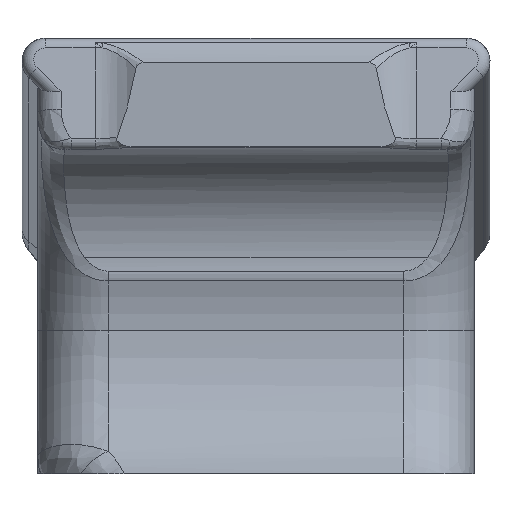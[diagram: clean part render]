
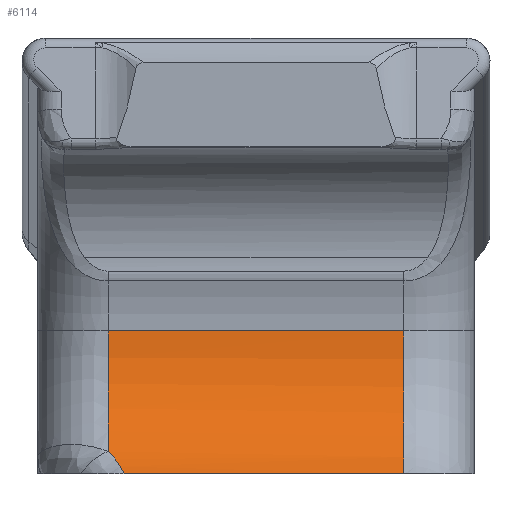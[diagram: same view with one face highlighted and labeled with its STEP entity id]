
A CAD part, left-side view. The second image highlights one B-rep face of the part: STEP entity #6114.
In plain terms, the highlighted cylindrical face has radius 14.287 mm (diameter 28.575 mm), a partial arc.
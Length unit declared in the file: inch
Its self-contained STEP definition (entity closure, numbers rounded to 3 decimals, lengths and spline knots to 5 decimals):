
#129 = CARTESIAN_POINT ( 'NONE',  ( 3.40993, -1.75491, -0.42132 ) ) ;
#167 = CARTESIAN_POINT ( 'NONE',  ( 3.33352, -1.80307, -0.48414 ) ) ;
#827 = B_SPLINE_CURVE_WITH_KNOTS ( 'NONE', 3,
 ( #129, #930, #6098, #1701, #6829, #2431, #7580, #3139, #8293, #3896, #9016, #4653, #167, #5401 ),
 .UNSPECIFIED., .F., .F.,
 ( 4, 2, 2, 1, 1, 2, 2, 4 ),
 ( 0., 0.25, 0.375, 0.4375, 0.46875, 0.48437, 0.5, 1. ),
 .UNSPECIFIED. ) ;
#930 = CARTESIAN_POINT ( 'NONE',  ( 3.40365, -1.76135, -0.42742 ) ) ;
#1022 = DIRECTION ( 'NONE',  ( 0., -1., 0. ) ) ;
#1089 = CARTESIAN_POINT ( 'NONE',  ( 3.31382, -2.74441, -0.49633 ) ) ;
#1487 = CARTESIAN_POINT ( 'NONE',  ( 3.31382, -1.80838, -0.49633 ) ) ;
#1536 = VECTOR ( 'NONE', #5245, 39.37008 ) ;
#1614 = LINE ( 'NONE', #5261, #1536 ) ;
#1629 = CIRCLE ( 'NONE', #3946, 0.5625 ) ;
#1701 = CARTESIAN_POINT ( 'NONE',  ( 3.386, -1.77556, -0.4433 ) ) ;
#1999 = CIRCLE ( 'NONE', #3565, 0.5625 ) ;
#2230 = VECTOR ( 'NONE', #1022, 39.37008 ) ;
#2263 = LINE ( 'NONE', #8339, #2230 ) ;
#2431 = CARTESIAN_POINT ( 'NONE',  ( 3.3764, -1.78195, -0.45141 ) ) ;
#2604 = EDGE_CURVE ( 'NONE', #6706, #9621, #2263, .T. ) ;
#2961 = EDGE_LOOP ( 'NONE', ( #6914, #5644, #6990, #7257, #7335 ) ) ;
#3139 = CARTESIAN_POINT ( 'NONE',  ( 3.36988, -1.78585, -0.45672 ) ) ;
#3213 = CYLINDRICAL_SURFACE ( 'NONE', #5020, 0.5625 ) ;
#3510 = CARTESIAN_POINT ( 'NONE',  ( 3.01782, -1.75491, -0.01801 ) ) ;
#3565 = AXIS2_PLACEMENT_3D ( 'NONE', #4063, #4031, #3993 ) ;
#3582 = EDGE_CURVE ( 'NONE', #6839, #8526, #1614, .T. ) ;
#3896 = CARTESIAN_POINT ( 'NONE',  ( 3.3673, -1.78729, -0.45877 ) ) ;
#3946 = AXIS2_PLACEMENT_3D ( 'NONE', #3510, #8634, #4250 ) ;
#3993 = DIRECTION ( 'NONE',  ( 1., 0., 0. ) ) ;
#4031 = DIRECTION ( 'NONE',  ( 0., -1., 0. ) ) ;
#4063 = CARTESIAN_POINT ( 'NONE',  ( 3.01782, -2.74441, -0.01801 ) ) ;
#4077 = CARTESIAN_POINT ( 'NONE',  ( 3.58032, -2.74441, -0.01801 ) ) ;
#4250 = DIRECTION ( 'NONE',  ( 1., 0., 0. ) ) ;
#4653 = CARTESIAN_POINT ( 'NONE',  ( 3.35092, -1.79623, -0.4717 ) ) ;
#4964 = VERTEX_POINT ( 'NONE', #5832 ) ;
#5020 = AXIS2_PLACEMENT_3D ( 'NONE', #8989, #7674, #7551 ) ;
#5245 = DIRECTION ( 'NONE',  ( 0., 1., 0. ) ) ;
#5261 = CARTESIAN_POINT ( 'NONE',  ( 3.58032, -2.81216, -0.01801 ) ) ;
#5401 = CARTESIAN_POINT ( 'NONE',  ( 3.31382, -1.80838, -0.49633 ) ) ;
#5579 = EDGE_CURVE ( 'NONE', #9621, #6839, #1999, .T. ) ;
#5644 = ORIENTED_EDGE ( 'NONE', *, *, #3582, .T. ) ;
#5832 = CARTESIAN_POINT ( 'NONE',  ( 3.40993, -1.75491, -0.42132 ) ) ;
#6098 = CARTESIAN_POINT ( 'NONE',  ( 3.3969, -1.76732, -0.4337 ) ) ;
#6114 = ADVANCED_FACE ( 'NONE', ( #9201 ), #3213, .F. ) ;
#6706 = VERTEX_POINT ( 'NONE', #1487 ) ;
#6829 = CARTESIAN_POINT ( 'NONE',  ( 3.38224, -1.77818, -0.44653 ) ) ;
#6839 = VERTEX_POINT ( 'NONE', #4077 ) ;
#6914 = ORIENTED_EDGE ( 'NONE', *, *, #5579, .T. ) ;
#6990 = ORIENTED_EDGE ( 'NONE', *, *, #8502, .T. ) ;
#7240 = EDGE_CURVE ( 'NONE', #4964, #6706, #827, .T. ) ;
#7257 = ORIENTED_EDGE ( 'NONE', *, *, #7240, .T. ) ;
#7335 = ORIENTED_EDGE ( 'NONE', *, *, #2604, .T. ) ;
#7551 = DIRECTION ( 'NONE',  ( 1., 0., 0. ) ) ;
#7580 = CARTESIAN_POINT ( 'NONE',  ( 3.37343, -1.78378, -0.45385 ) ) ;
#7674 = DIRECTION ( 'NONE',  ( 0., 1., 0. ) ) ;
#7921 = CARTESIAN_POINT ( 'NONE',  ( 3.58032, -1.75491, -0.01801 ) ) ;
#8293 = CARTESIAN_POINT ( 'NONE',  ( 3.36833, -1.78672, -0.45795 ) ) ;
#8339 = CARTESIAN_POINT ( 'NONE',  ( 3.31382, -2.81216, -0.49633 ) ) ;
#8502 = EDGE_CURVE ( 'NONE', #8526, #4964, #1629, .T. ) ;
#8526 = VERTEX_POINT ( 'NONE', #7921 ) ;
#8634 = DIRECTION ( 'NONE',  ( 0., 1., 0. ) ) ;
#8989 = CARTESIAN_POINT ( 'NONE',  ( 3.01782, -2.81216, -0.01801 ) ) ;
#9016 = CARTESIAN_POINT ( 'NONE',  ( 3.36674, -1.7876, -0.45921 ) ) ;
#9201 = FACE_OUTER_BOUND ( 'NONE', #2961, .T. ) ;
#9621 = VERTEX_POINT ( 'NONE', #1089 ) ;
